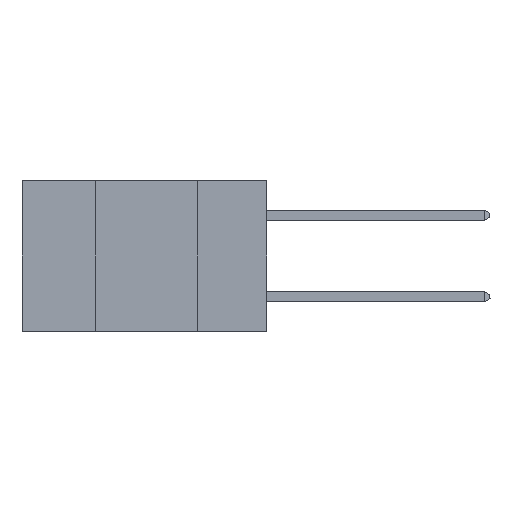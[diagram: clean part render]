
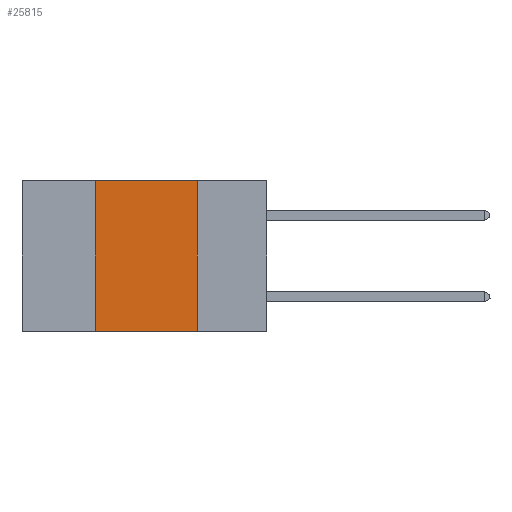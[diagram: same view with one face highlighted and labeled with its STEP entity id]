
A CAD part, left-side view. The second image highlights one B-rep face of the part: STEP entity #25815.
In plain terms, the highlighted planar face has unit normal (-1, 0, 0).
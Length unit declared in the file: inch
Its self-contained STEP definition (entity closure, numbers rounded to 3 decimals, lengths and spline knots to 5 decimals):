
#134 = AXIS2_PLACEMENT_3D ( 'NONE', #9873, #19915, #42065 ) ;
#1922 = VERTEX_POINT ( 'NONE', #22201 ) ;
#4539 = FACE_OUTER_BOUND ( 'NONE', #9341, .T. ) ;
#4696 = EDGE_CURVE ( 'NONE', #23719, #1922, #12832, .T. ) ;
#5874 = DIRECTION ( 'NONE',  ( 0., -1., 0. ) ) ;
#7061 = DIRECTION ( 'NONE',  ( 0., 0., 1. ) ) ;
#8924 = CARTESIAN_POINT ( 'NONE',  ( 0., 0.6, 0. ) ) ;
#9197 = LINE ( 'NONE', #23592, #25668 ) ;
#9341 = EDGE_LOOP ( 'NONE', ( #33421, #17441, #10628, #13797 ) ) ;
#9873 = CARTESIAN_POINT ( 'NONE',  ( 0., 0.6, 0. ) ) ;
#10044 = EDGE_CURVE ( 'NONE', #19969, #33073, #9197, .T. ) ;
#10628 = ORIENTED_EDGE ( 'NONE', *, *, #10044, .F. ) ;
#12832 = LINE ( 'NONE', #18454, #29105 ) ;
#13797 = ORIENTED_EDGE ( 'NONE', *, *, #35026, .T. ) ;
#17441 = ORIENTED_EDGE ( 'NONE', *, *, #20954, .F. ) ;
#18454 = CARTESIAN_POINT ( 'NONE',  ( 0., 0.17, 0. ) ) ;
#19915 = DIRECTION ( 'NONE',  ( 1., 0., 0. ) ) ;
#19969 = VERTEX_POINT ( 'NONE', #36144 ) ;
#20305 = VECTOR ( 'NONE', #5874, 39.37008 ) ;
#20954 = EDGE_CURVE ( 'NONE', #33073, #23719, #33515, .T. ) ;
#22201 = CARTESIAN_POINT ( 'NONE',  ( 0., 0.17, -0.37 ) ) ;
#23592 = CARTESIAN_POINT ( 'NONE',  ( 0., 0.42, 0. ) ) ;
#23719 = VERTEX_POINT ( 'NONE', #25774 ) ;
#24174 = VECTOR ( 'NONE', #28534, 39.37008 ) ;
#25659 = CARTESIAN_POINT ( 'NONE',  ( 0., 0.6, -0.37 ) ) ;
#25668 = VECTOR ( 'NONE', #7061, 39.37008 ) ;
#25774 = CARTESIAN_POINT ( 'NONE',  ( 0., 0.17, 0. ) ) ;
#25815 = ADVANCED_FACE ( 'NONE', ( #4539 ), #38875, .F. ) ;
#27825 = LINE ( 'NONE', #25659, #20305 ) ;
#28534 = DIRECTION ( 'NONE',  ( 0., -1., 0. ) ) ;
#29105 = VECTOR ( 'NONE', #37476, 39.37008 ) ;
#33039 = CARTESIAN_POINT ( 'NONE',  ( 0., 0.42, 0. ) ) ;
#33073 = VERTEX_POINT ( 'NONE', #33039 ) ;
#33421 = ORIENTED_EDGE ( 'NONE', *, *, #4696, .F. ) ;
#33515 = LINE ( 'NONE', #8924, #24174 ) ;
#35026 = EDGE_CURVE ( 'NONE', #19969, #1922, #27825, .T. ) ;
#36144 = CARTESIAN_POINT ( 'NONE',  ( 0., 0.42, -0.37 ) ) ;
#37476 = DIRECTION ( 'NONE',  ( 0., 0., -1. ) ) ;
#38875 = PLANE ( 'NONE',  #134 ) ;
#42065 = DIRECTION ( 'NONE',  ( 0., 0., -1. ) ) ;
